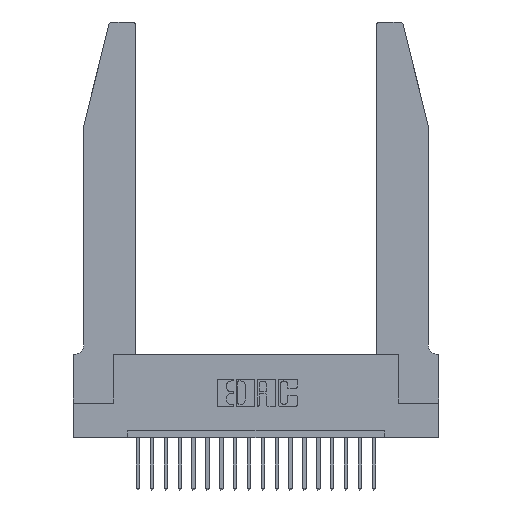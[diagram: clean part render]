
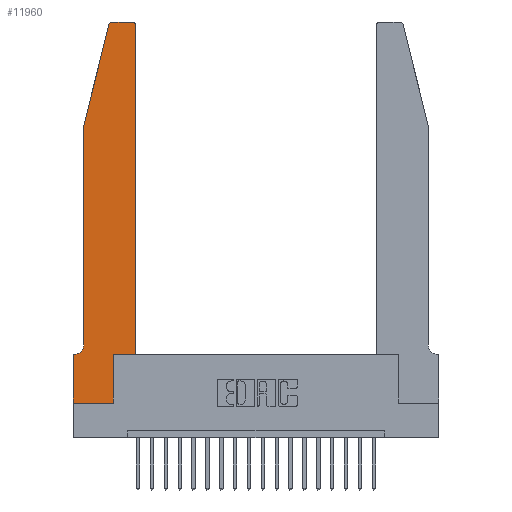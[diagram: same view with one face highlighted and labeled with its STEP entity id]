
A CAD part, top view. The second image highlights one B-rep face of the part: STEP entity #11960.
In plain terms, the highlighted planar face has unit normal (0, 0, 1).
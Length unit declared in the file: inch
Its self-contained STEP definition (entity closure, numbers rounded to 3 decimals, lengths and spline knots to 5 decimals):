
#39 = LINE ( 'NONE', #13500, #5273 ) ;
#168 = DIRECTION ( 'NONE',  ( 0., 0., 1. ) ) ;
#289 = DIRECTION ( 'NONE',  ( 0., 1., 0. ) ) ;
#358 = LINE ( 'NONE', #15871, #8748 ) ;
#419 = CARTESIAN_POINT ( 'NONE',  ( 0.284, 2.75, 0.37 ) ) ;
#686 = CIRCLE ( 'NONE', #7527, 0.03 ) ;
#729 = LINE ( 'NONE', #3385, #19488 ) ;
#772 = EDGE_CURVE ( 'NONE', #10488, #10979, #9468, .T. ) ;
#814 = CIRCLE ( 'NONE', #2027, 0.03 ) ;
#1235 = DIRECTION ( 'NONE',  ( -0.239, -0.971, 0. ) ) ;
#1983 = EDGE_CURVE ( 'NONE', #10942, #12388, #39, .T. ) ;
#2027 = AXIS2_PLACEMENT_3D ( 'NONE', #16843, #11114, #20189 ) ;
#2303 = CARTESIAN_POINT ( 'NONE',  ( 0.0055, 0.42, 0.37 ) ) ;
#2566 = VECTOR ( 'NONE', #6693, 39.37008 ) ;
#3280 = VECTOR ( 'NONE', #18617, 39.37008 ) ;
#3385 = CARTESIAN_POINT ( 'NONE',  ( 0., 0., 0.37 ) ) ;
#3449 = ORIENTED_EDGE ( 'NONE', *, *, #21314, .T. ) ;
#3453 = EDGE_CURVE ( 'NONE', #13026, #10942, #729, .T. ) ;
#3532 = DIRECTION ( 'NONE',  ( 1., 0., 0. ) ) ;
#3646 = LINE ( 'NONE', #13231, #4707 ) ;
#3676 = ORIENTED_EDGE ( 'NONE', *, *, #6004, .T. ) ;
#3837 = DIRECTION ( 'NONE',  ( 0., -1., 0. ) ) ;
#4065 = DIRECTION ( 'NONE',  ( 0., 0., -1. ) ) ;
#4221 = VERTEX_POINT ( 'NONE', #15982 ) ;
#4452 = CARTESIAN_POINT ( 'NONE',  ( 0.2605, 2.75, 0.37 ) ) ;
#4468 = CARTESIAN_POINT ( 'NONE',  ( 0., 0., 0.37 ) ) ;
#4480 = ORIENTED_EDGE ( 'NONE', *, *, #8150, .T. ) ;
#4599 = EDGE_CURVE ( 'NONE', #11656, #20900, #686, .T. ) ;
#4658 = VECTOR ( 'NONE', #3837, 39.37008 ) ;
#4707 = VECTOR ( 'NONE', #6639, 39.37008 ) ;
#5273 = VECTOR ( 'NONE', #289, 39.37008 ) ;
#5781 = ORIENTED_EDGE ( 'NONE', *, *, #20410, .T. ) ;
#6004 = EDGE_CURVE ( 'NONE', #12291, #4221, #358, .T. ) ;
#6068 = ORIENTED_EDGE ( 'NONE', *, *, #17658, .T. ) ;
#6105 = ORIENTED_EDGE ( 'NONE', *, *, #3453, .T. ) ;
#6431 = LINE ( 'NONE', #13570, #3280 ) ;
#6639 = DIRECTION ( 'NONE',  ( 1., 0., 0. ) ) ;
#6693 = DIRECTION ( 'NONE',  ( -1., 0., 0. ) ) ;
#7527 = AXIS2_PLACEMENT_3D ( 'NONE', #11784, #168, #13519 ) ;
#7565 = CARTESIAN_POINT ( 'NONE',  ( 0.0755, 0.35, 0.37 ) ) ;
#8007 = EDGE_CURVE ( 'NONE', #9665, #11656, #20848, .T. ) ;
#8150 = EDGE_CURVE ( 'NONE', #4221, #9665, #814, .T. ) ;
#8211 = CARTESIAN_POINT ( 'NONE',  ( 0.25487, 2.72718, 0.37 ) ) ;
#8748 = VECTOR ( 'NONE', #10486, 39.37008 ) ;
#8950 = CARTESIAN_POINT ( 'NONE',  ( 0.0755, 2., 0.37 ) ) ;
#9062 = EDGE_LOOP ( 'NONE', ( #16580, #20243, #3449, #16877, #13210, #6068, #5781, #6105, #9530, #13312, #3676, #4480 ) ) ;
#9065 = EDGE_CURVE ( 'NONE', #17367, #10488, #15080, .T. ) ;
#9468 = CIRCLE ( 'NONE', #17633, 0.07 ) ;
#9520 = VECTOR ( 'NONE', #1235, 39.37008 ) ;
#9530 = ORIENTED_EDGE ( 'NONE', *, *, #1983, .T. ) ;
#9533 = CARTESIAN_POINT ( 'NONE',  ( 0.4505, 0.35, 0.37 ) ) ;
#9665 = VERTEX_POINT ( 'NONE', #10126 ) ;
#10047 = LINE ( 'NONE', #16225, #9520 ) ;
#10126 = CARTESIAN_POINT ( 'NONE',  ( 0.4205, 2.75, 0.37 ) ) ;
#10347 = CARTESIAN_POINT ( 'NONE',  ( 0., 0.35, 0.37 ) ) ;
#10486 = DIRECTION ( 'NONE',  ( 0., 1., 0. ) ) ;
#10488 = VERTEX_POINT ( 'NONE', #13992 ) ;
#10942 = VERTEX_POINT ( 'NONE', #13906 ) ;
#10979 = VERTEX_POINT ( 'NONE', #15776 ) ;
#11114 = DIRECTION ( 'NONE',  ( 0., 0., 1. ) ) ;
#11474 = CARTESIAN_POINT ( 'NONE',  ( 0.2865, 0.35, 0.37 ) ) ;
#11656 = VERTEX_POINT ( 'NONE', #419 ) ;
#11784 = CARTESIAN_POINT ( 'NONE',  ( 0.284, 2.72, 0.37 ) ) ;
#11960 = ADVANCED_FACE ( 'NONE', ( #13123 ), #14103, .T. ) ;
#11984 = AXIS2_PLACEMENT_3D ( 'NONE', #14315, #15894, #15819 ) ;
#12291 = VERTEX_POINT ( 'NONE', #9533 ) ;
#12388 = VERTEX_POINT ( 'NONE', #11474 ) ;
#13026 = VERTEX_POINT ( 'NONE', #4468 ) ;
#13079 = DIRECTION ( 'NONE',  ( -1., 0., 0. ) ) ;
#13123 = FACE_OUTER_BOUND ( 'NONE', #9062, .T. ) ;
#13210 = ORIENTED_EDGE ( 'NONE', *, *, #772, .T. ) ;
#13231 = CARTESIAN_POINT ( 'NONE',  ( 0.4505, 0.35, 0.37 ) ) ;
#13312 = ORIENTED_EDGE ( 'NONE', *, *, #17185, .T. ) ;
#13500 = CARTESIAN_POINT ( 'NONE',  ( 0.2865, 0.35, 0.37 ) ) ;
#13519 = DIRECTION ( 'NONE',  ( 1., 0., 0. ) ) ;
#13570 = CARTESIAN_POINT ( 'NONE',  ( 0., 0., 0.37 ) ) ;
#13906 = CARTESIAN_POINT ( 'NONE',  ( 0.2865, 0., 0.37 ) ) ;
#13992 = CARTESIAN_POINT ( 'NONE',  ( 0.0755, 0.42, 0.37 ) ) ;
#14103 = PLANE ( 'NONE',  #11984 ) ;
#14315 = CARTESIAN_POINT ( 'NONE',  ( 0., 0.35, 0.37 ) ) ;
#14587 = LINE ( 'NONE', #7565, #2566 ) ;
#15080 = LINE ( 'NONE', #8950, #4658 ) ;
#15415 = VECTOR ( 'NONE', #13079, 39.37008 ) ;
#15626 = DIRECTION ( 'NONE',  ( -1., 0., 0. ) ) ;
#15776 = CARTESIAN_POINT ( 'NONE',  ( 0.0055, 0.35, 0.37 ) ) ;
#15819 = DIRECTION ( 'NONE',  ( 1., 0., 0. ) ) ;
#15871 = CARTESIAN_POINT ( 'NONE',  ( 0.4505, 0.35, 0.37 ) ) ;
#15894 = DIRECTION ( 'NONE',  ( 0., 0., 1. ) ) ;
#15982 = CARTESIAN_POINT ( 'NONE',  ( 0.4505, 2.72, 0.37 ) ) ;
#16225 = CARTESIAN_POINT ( 'NONE',  ( 0.0755, 2., 0.37 ) ) ;
#16580 = ORIENTED_EDGE ( 'NONE', *, *, #8007, .T. ) ;
#16843 = CARTESIAN_POINT ( 'NONE',  ( 0.4205, 2.72, 0.37 ) ) ;
#16877 = ORIENTED_EDGE ( 'NONE', *, *, #9065, .T. ) ;
#16929 = CARTESIAN_POINT ( 'NONE',  ( 0.0755, 2., 0.37 ) ) ;
#17185 = EDGE_CURVE ( 'NONE', #12388, #12291, #3646, .T. ) ;
#17367 = VERTEX_POINT ( 'NONE', #16929 ) ;
#17633 = AXIS2_PLACEMENT_3D ( 'NONE', #2303, #4065, #15626 ) ;
#17658 = EDGE_CURVE ( 'NONE', #10979, #19233, #14587, .T. ) ;
#18617 = DIRECTION ( 'NONE',  ( 0., -1., 0. ) ) ;
#19233 = VERTEX_POINT ( 'NONE', #10347 ) ;
#19488 = VECTOR ( 'NONE', #3532, 39.37008 ) ;
#20189 = DIRECTION ( 'NONE',  ( 1., 0., 0. ) ) ;
#20243 = ORIENTED_EDGE ( 'NONE', *, *, #4599, .T. ) ;
#20410 = EDGE_CURVE ( 'NONE', #19233, #13026, #6431, .T. ) ;
#20848 = LINE ( 'NONE', #4452, #15415 ) ;
#20900 = VERTEX_POINT ( 'NONE', #8211 ) ;
#21314 = EDGE_CURVE ( 'NONE', #20900, #17367, #10047, .T. ) ;
